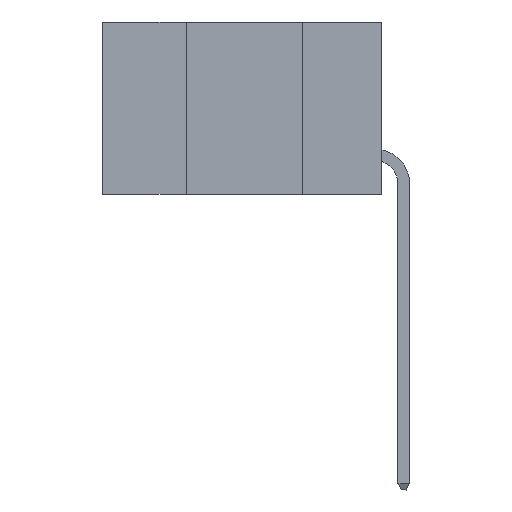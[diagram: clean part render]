
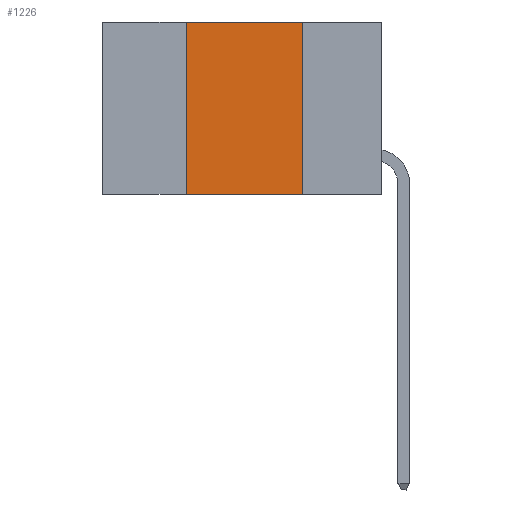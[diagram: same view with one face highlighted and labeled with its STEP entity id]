
A CAD part, left-side view. The second image highlights one B-rep face of the part: STEP entity #1226.
In plain terms, the highlighted planar face has unit normal (-1, 0, 0).
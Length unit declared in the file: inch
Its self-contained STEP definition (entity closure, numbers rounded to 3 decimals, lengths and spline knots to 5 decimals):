
#47 = EDGE_CURVE ( 'NONE', #9116, #3555, #1061, .T. ) ;
#253 = EDGE_CURVE ( 'NONE', #9116, #5669, #3704, .T. ) ;
#263 = CARTESIAN_POINT ( 'NONE',  ( 0., 0.42, -0.37 ) ) ;
#366 = VECTOR ( 'NONE', #6386, 39.37008 ) ;
#421 = EDGE_CURVE ( 'NONE', #6413, #3555, #6376, .T. ) ;
#782 = VECTOR ( 'NONE', #6415, 39.37008 ) ;
#784 = FACE_OUTER_BOUND ( 'NONE', #1431, .T. ) ;
#1061 = LINE ( 'NONE', #3254, #366 ) ;
#1178 = CARTESIAN_POINT ( 'NONE',  ( 0., 0.6, 0. ) ) ;
#1226 = ADVANCED_FACE ( 'NONE', ( #784 ), #2402, .F. ) ;
#1431 = EDGE_LOOP ( 'NONE', ( #2700, #6256, #9219, #5889 ) ) ;
#1749 = DIRECTION ( 'NONE',  ( 0., -1., 0. ) ) ;
#2402 = PLANE ( 'NONE',  #6827 ) ;
#2700 = ORIENTED_EDGE ( 'NONE', *, *, #421, .F. ) ;
#3095 = VECTOR ( 'NONE', #1749, 39.37008 ) ;
#3254 = CARTESIAN_POINT ( 'NONE',  ( 0., 0.6, -0.37 ) ) ;
#3263 = VECTOR ( 'NONE', #9274, 39.37008 ) ;
#3555 = VERTEX_POINT ( 'NONE', #6191 ) ;
#3704 = LINE ( 'NONE', #5956, #3263 ) ;
#3989 = CARTESIAN_POINT ( 'NONE',  ( 0., 0.6, 0. ) ) ;
#4114 = CARTESIAN_POINT ( 'NONE',  ( 0., 0.42, 0. ) ) ;
#5604 = CARTESIAN_POINT ( 'NONE',  ( 0., 0.17, 0. ) ) ;
#5669 = VERTEX_POINT ( 'NONE', #4114 ) ;
#5889 = ORIENTED_EDGE ( 'NONE', *, *, #47, .T. ) ;
#5956 = CARTESIAN_POINT ( 'NONE',  ( 0., 0.42, 0. ) ) ;
#6191 = CARTESIAN_POINT ( 'NONE',  ( 0., 0.17, -0.37 ) ) ;
#6195 = DIRECTION ( 'NONE',  ( 1., 0., 0. ) ) ;
#6256 = ORIENTED_EDGE ( 'NONE', *, *, #7032, .F. ) ;
#6376 = LINE ( 'NONE', #5604, #782 ) ;
#6386 = DIRECTION ( 'NONE',  ( 0., -1., 0. ) ) ;
#6413 = VERTEX_POINT ( 'NONE', #9289 ) ;
#6415 = DIRECTION ( 'NONE',  ( 0., 0., -1. ) ) ;
#6827 = AXIS2_PLACEMENT_3D ( 'NONE', #3989, #6195, #9404 ) ;
#7032 = EDGE_CURVE ( 'NONE', #5669, #6413, #7192, .T. ) ;
#7192 = LINE ( 'NONE', #1178, #3095 ) ;
#9116 = VERTEX_POINT ( 'NONE', #263 ) ;
#9219 = ORIENTED_EDGE ( 'NONE', *, *, #253, .F. ) ;
#9274 = DIRECTION ( 'NONE',  ( 0., 0., 1. ) ) ;
#9289 = CARTESIAN_POINT ( 'NONE',  ( 0., 0.17, 0. ) ) ;
#9404 = DIRECTION ( 'NONE',  ( 0., 0., -1. ) ) ;
